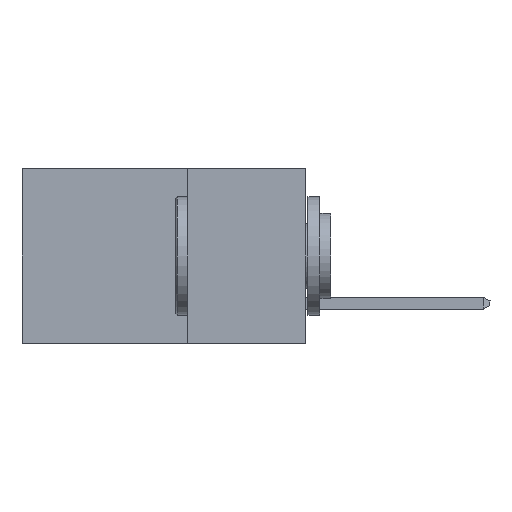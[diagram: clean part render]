
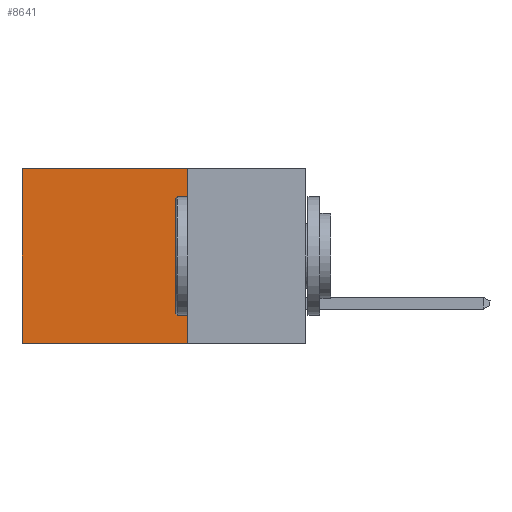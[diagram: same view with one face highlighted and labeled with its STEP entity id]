
A CAD part, left-side view. The second image highlights one B-rep face of the part: STEP entity #8641.
In plain terms, the highlighted planar face has unit normal (-1, 0, 0).
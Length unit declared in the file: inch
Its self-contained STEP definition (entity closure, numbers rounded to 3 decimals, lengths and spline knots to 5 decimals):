
#866 = CARTESIAN_POINT ( 'NONE',  ( 0.298, 0.6, 0. ) ) ;
#2350 = CARTESIAN_POINT ( 'NONE',  ( 0.298, 0.25, 0. ) ) ;
#2717 = EDGE_CURVE ( 'NONE', #3745, #6770, #4359, .T. ) ;
#3745 = VERTEX_POINT ( 'NONE', #2350 ) ;
#4359 = LINE ( 'NONE', #5945, #14817 ) ;
#4805 = CARTESIAN_POINT ( 'NONE',  ( 0.298, 0.6, 0. ) ) ;
#5873 = VECTOR ( 'NONE', #14982, 39.37008 ) ;
#5945 = CARTESIAN_POINT ( 'NONE',  ( 0.298, 0.25, 0. ) ) ;
#6078 = LINE ( 'NONE', #866, #11670 ) ;
#6770 = VERTEX_POINT ( 'NONE', #4805 ) ;
#7556 = DIRECTION ( 'NONE',  ( 0., 0., -1. ) ) ;
#8192 = DIRECTION ( 'NONE',  ( 0., 1., 0. ) ) ;
#8641 = ADVANCED_FACE ( 'NONE', ( #9220 ), #12333, .F. ) ;
#8718 = AXIS2_PLACEMENT_3D ( 'NONE', #21186, #21097, #7556 ) ;
#8754 = EDGE_CURVE ( 'NONE', #6770, #19311, #6078, .T. ) ;
#8918 = CARTESIAN_POINT ( 'NONE',  ( 0.298, 0.25, -0.37 ) ) ;
#9220 = FACE_OUTER_BOUND ( 'NONE', #12098, .T. ) ;
#10940 = ORIENTED_EDGE ( 'NONE', *, *, #27648, .F. ) ;
#10965 = VECTOR ( 'NONE', #25976, 39.37008 ) ;
#11670 = VECTOR ( 'NONE', #18693, 39.37008 ) ;
#12098 = EDGE_LOOP ( 'NONE', ( #24517, #26729, #10940, #21394 ) ) ;
#12333 = PLANE ( 'NONE',  #8718 ) ;
#12946 = CARTESIAN_POINT ( 'NONE',  ( 0.298, 0.25, -0.37 ) ) ;
#14817 = VECTOR ( 'NONE', #8192, 39.37008 ) ;
#14982 = DIRECTION ( 'NONE',  ( 0., 1., 0. ) ) ;
#17424 = CARTESIAN_POINT ( 'NONE',  ( 0.298, 0.25, 0. ) ) ;
#18693 = DIRECTION ( 'NONE',  ( 0., 0., -1. ) ) ;
#19311 = VERTEX_POINT ( 'NONE', #21320 ) ;
#21097 = DIRECTION ( 'NONE',  ( 1., 0., 0. ) ) ;
#21186 = CARTESIAN_POINT ( 'NONE',  ( 0.298, 0.25, 0. ) ) ;
#21320 = CARTESIAN_POINT ( 'NONE',  ( 0.298, 0.6, -0.37 ) ) ;
#21394 = ORIENTED_EDGE ( 'NONE', *, *, #2717, .T. ) ;
#22963 = LINE ( 'NONE', #8918, #5873 ) ;
#23272 = VERTEX_POINT ( 'NONE', #12946 ) ;
#24517 = ORIENTED_EDGE ( 'NONE', *, *, #8754, .T. ) ;
#24528 = LINE ( 'NONE', #17424, #10965 ) ;
#25411 = EDGE_CURVE ( 'NONE', #23272, #19311, #22963, .T. ) ;
#25976 = DIRECTION ( 'NONE',  ( 0., 0., -1. ) ) ;
#26729 = ORIENTED_EDGE ( 'NONE', *, *, #25411, .F. ) ;
#27648 = EDGE_CURVE ( 'NONE', #3745, #23272, #24528, .T. ) ;
